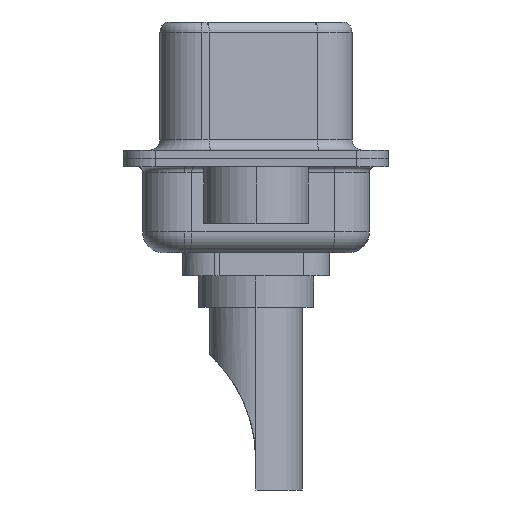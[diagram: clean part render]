
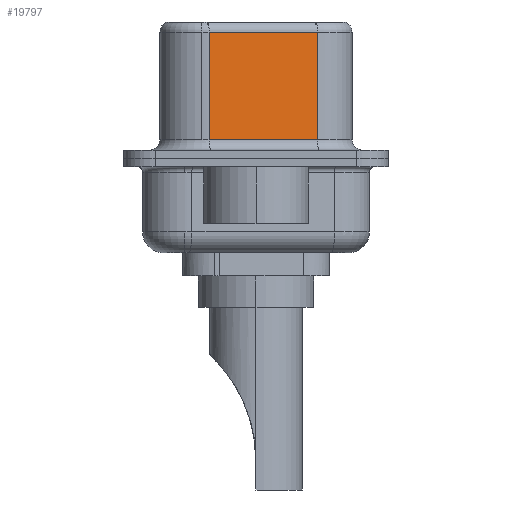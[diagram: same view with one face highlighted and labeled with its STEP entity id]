
A CAD part, left-side view. The second image highlights one B-rep face of the part: STEP entity #19797.
In plain terms, the highlighted planar face has unit normal (-0.985, -0.174, 0).
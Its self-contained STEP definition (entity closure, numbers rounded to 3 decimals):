
#1262 = VECTOR ( 'NONE', #22947, 1000. ) ;
#1544 = EDGE_CURVE ( 'NONE', #17976, #17986, #9533, .T. ) ;
#1553 = EDGE_LOOP ( 'NONE', ( #11273, #22877, #20972, #5884 ) ) ;
#2456 = LINE ( 'NONE', #21017, #1262 ) ;
#2570 = CARTESIAN_POINT ( 'NONE',  ( 4.58, -2.927, 0.9 ) ) ;
#3698 = CARTESIAN_POINT ( 'NONE',  ( 4.58, -2.927, 6.52 ) ) ;
#4220 = DIRECTION ( 'NONE',  ( -0.174, 0.985, 0. ) ) ;
#5884 = ORIENTED_EDGE ( 'NONE', *, *, #13490, .T. ) ;
#6428 = DIRECTION ( 'NONE',  ( 0.174, -0.985, 0. ) ) ;
#7324 = DIRECTION ( 'NONE',  ( 0., 0., -1. ) ) ;
#9108 = LINE ( 'NONE', #2570, #23032 ) ;
#9436 = PLANE ( 'NONE',  #18937 ) ;
#9533 = LINE ( 'NONE', #15697, #14551 ) ;
#11273 = ORIENTED_EDGE ( 'NONE', *, *, #1544, .F. ) ;
#11369 = DIRECTION ( 'NONE',  ( -0.174, 0.985, 0. ) ) ;
#12008 = VERTEX_POINT ( 'NONE', #19496 ) ;
#12416 = LINE ( 'NONE', #19285, #16836 ) ;
#13490 = EDGE_CURVE ( 'NONE', #12008, #17986, #9108, .T. ) ;
#13868 = EDGE_CURVE ( 'NONE', #17976, #15986, #12416, .T. ) ;
#14551 = VECTOR ( 'NONE', #7324, 1000. ) ;
#15697 = CARTESIAN_POINT ( 'NONE',  ( 4.58, -2.927, 6.52 ) ) ;
#15986 = VERTEX_POINT ( 'NONE', #19191 ) ;
#16004 = CARTESIAN_POINT ( 'NONE',  ( 4.58, -2.927, 0.9 ) ) ;
#16836 = VECTOR ( 'NONE', #4220, 1000. ) ;
#17832 = CARTESIAN_POINT ( 'NONE',  ( 4.58, -2.927, 6.02 ) ) ;
#17976 = VERTEX_POINT ( 'NONE', #17832 ) ;
#17986 = VERTEX_POINT ( 'NONE', #16004 ) ;
#18937 = AXIS2_PLACEMENT_3D ( 'NONE', #3698, #22664, #11369 ) ;
#19191 = CARTESIAN_POINT ( 'NONE',  ( 3.67, 2.233, 6.02 ) ) ;
#19285 = CARTESIAN_POINT ( 'NONE',  ( 4.58, -2.927, 6.02 ) ) ;
#19496 = CARTESIAN_POINT ( 'NONE',  ( 3.67, 2.233, 0.9 ) ) ;
#19797 = ADVANCED_FACE ( 'NONE', ( #21519 ), #9436, .F. ) ;
#20972 = ORIENTED_EDGE ( 'NONE', *, *, #22065, .T. ) ;
#21017 = CARTESIAN_POINT ( 'NONE',  ( 3.67, 2.233, 6.52 ) ) ;
#21519 = FACE_OUTER_BOUND ( 'NONE', #1553, .T. ) ;
#22065 = EDGE_CURVE ( 'NONE', #15986, #12008, #2456, .T. ) ;
#22664 = DIRECTION ( 'NONE',  ( 0.985, 0.174, 0. ) ) ;
#22877 = ORIENTED_EDGE ( 'NONE', *, *, #13868, .T. ) ;
#22947 = DIRECTION ( 'NONE',  ( 0., 0., -1. ) ) ;
#23032 = VECTOR ( 'NONE', #6428, 1000. ) ;
